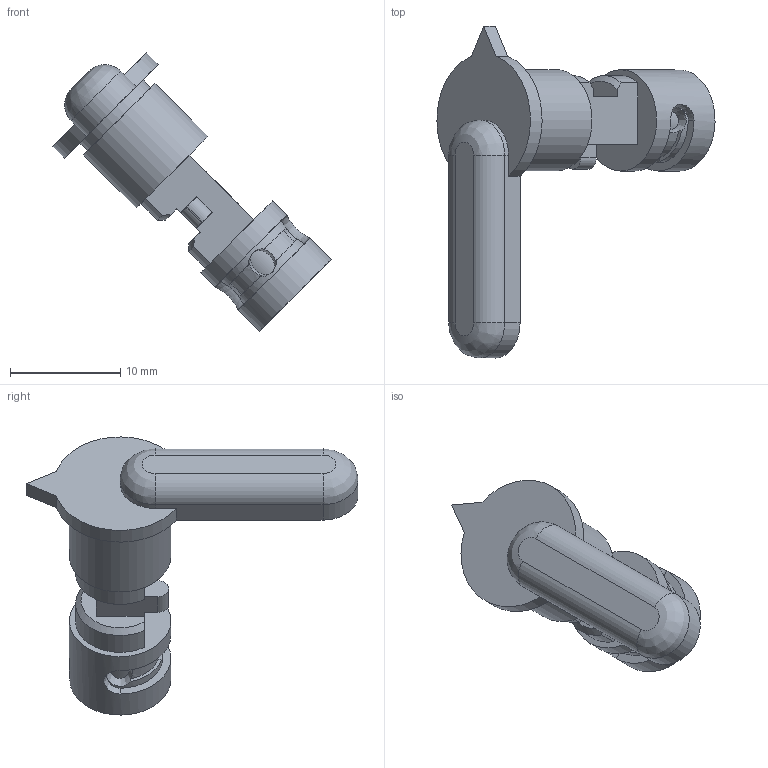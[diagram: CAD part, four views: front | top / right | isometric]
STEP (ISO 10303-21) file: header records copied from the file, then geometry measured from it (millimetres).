
FILE_DESCRIPTION(/* description */ (''),/* implementation_level */ '2;1');
FILE_NAME(/* name */ '',/* time_stamp */ '2021-12-08T23:02:38-05:00',/* author */ (''),/* organization */ (''),/* preprocessor_version */ 'ST-DEVELOPER v18.1',/* originating_system */ 'Autodesk Inventor 2022',/* authorisation */ '');
FILE_SCHEMA (('AUTOMOTIVE_DESIGN { 1 0 10303 214 3 1 1 }'));
Length unit declared in the file: inch
Products named in the file (1): YBS2 SS
Bounding box: 25.24 x 30.13 x 25.24 mm (x, y, z)
Volume: 1788.9 mm3; surface area: 1401.5 mm2
Topology: 1 solids, 1 shells, 62 faces, 159 edges, 104 vertices
Faces by surface type: plane 31, cylinder 21, bspline 7, cone 3
Full cylindrical faces by diameter (mm): 8.1 x1, 9.2 x2
Entity records: 2436 total; most frequent: CARTESIAN_POINT 878, ORIENTED_EDGE 318, DIRECTION 302, EDGE_CURVE 159, AXIS2_PLACEMENT_3D 113, VERTEX_POINT 104, LINE 76, VECTOR 76
